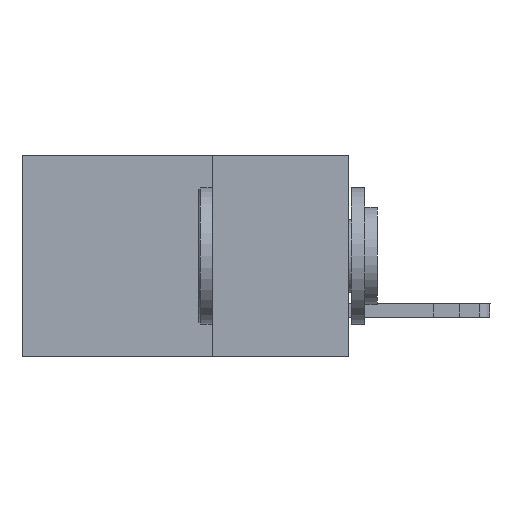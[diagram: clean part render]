
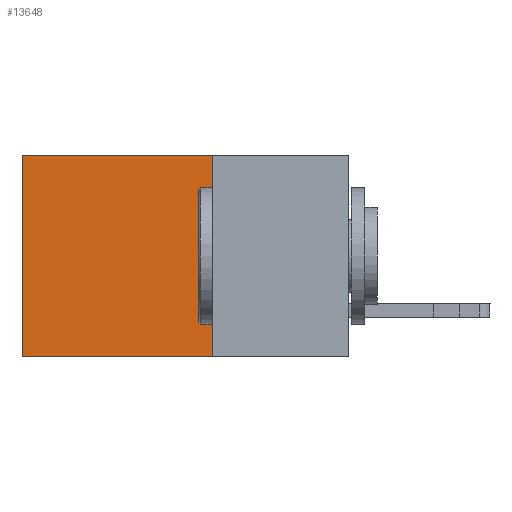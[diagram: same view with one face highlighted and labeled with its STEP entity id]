
A CAD part, left-side view. The second image highlights one B-rep face of the part: STEP entity #13648.
In plain terms, the highlighted planar face has unit normal (-1, 0, 0).
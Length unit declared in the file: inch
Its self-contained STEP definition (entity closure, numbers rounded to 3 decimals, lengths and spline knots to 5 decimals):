
#90 = VERTEX_POINT ( 'NONE', #14742 ) ;
#517 = LINE ( 'NONE', #11431, #14015 ) ;
#1959 = DIRECTION ( 'NONE',  ( 0., 0., -1. ) ) ;
#2169 = FACE_OUTER_BOUND ( 'NONE', #11980, .T. ) ;
#3057 = CARTESIAN_POINT ( 'NONE',  ( 0.298, 0.25, 0. ) ) ;
#3629 = VERTEX_POINT ( 'NONE', #11066 ) ;
#4095 = AXIS2_PLACEMENT_3D ( 'NONE', #15564, #9477, #11961 ) ;
#4279 = VECTOR ( 'NONE', #1959, 39.37008 ) ;
#5092 = VERTEX_POINT ( 'NONE', #12670 ) ;
#5637 = CARTESIAN_POINT ( 'NONE',  ( 0.298, 0.25, -0.37 ) ) ;
#6116 = ORIENTED_EDGE ( 'NONE', *, *, #13691, .F. ) ;
#6159 = VERTEX_POINT ( 'NONE', #5637 ) ;
#7059 = PLANE ( 'NONE',  #4095 ) ;
#7241 = EDGE_CURVE ( 'NONE', #6159, #3629, #517, .T. ) ;
#7521 = DIRECTION ( 'NONE',  ( 0., 0., -1. ) ) ;
#8971 = ORIENTED_EDGE ( 'NONE', *, *, #7241, .F. ) ;
#9103 = DIRECTION ( 'NONE',  ( 0., 1., 0. ) ) ;
#9477 = DIRECTION ( 'NONE',  ( 1., 0., 0. ) ) ;
#9647 = ORIENTED_EDGE ( 'NONE', *, *, #14740, .T. ) ;
#9884 = EDGE_CURVE ( 'NONE', #90, #3629, #15367, .T. ) ;
#10474 = CARTESIAN_POINT ( 'NONE',  ( 0.298, 0.6, 0. ) ) ;
#11066 = CARTESIAN_POINT ( 'NONE',  ( 0.298, 0.6, -0.37 ) ) ;
#11431 = CARTESIAN_POINT ( 'NONE',  ( 0.298, 0.25, -0.37 ) ) ;
#11881 = DIRECTION ( 'NONE',  ( 0., 1., 0. ) ) ;
#11961 = DIRECTION ( 'NONE',  ( 0., 0., -1. ) ) ;
#11980 = EDGE_LOOP ( 'NONE', ( #12576, #8971, #6116, #9647 ) ) ;
#12508 = LINE ( 'NONE', #13483, #15358 ) ;
#12576 = ORIENTED_EDGE ( 'NONE', *, *, #9884, .T. ) ;
#12670 = CARTESIAN_POINT ( 'NONE',  ( 0.298, 0.25, 0. ) ) ;
#13350 = VECTOR ( 'NONE', #11881, 39.37008 ) ;
#13483 = CARTESIAN_POINT ( 'NONE',  ( 0.298, 0.25, 0. ) ) ;
#13648 = ADVANCED_FACE ( 'NONE', ( #2169 ), #7059, .F. ) ;
#13691 = EDGE_CURVE ( 'NONE', #5092, #6159, #12508, .T. ) ;
#14015 = VECTOR ( 'NONE', #9103, 39.37008 ) ;
#14052 = LINE ( 'NONE', #3057, #13350 ) ;
#14740 = EDGE_CURVE ( 'NONE', #5092, #90, #14052, .T. ) ;
#14742 = CARTESIAN_POINT ( 'NONE',  ( 0.298, 0.6, 0. ) ) ;
#15358 = VECTOR ( 'NONE', #7521, 39.37008 ) ;
#15367 = LINE ( 'NONE', #10474, #4279 ) ;
#15564 = CARTESIAN_POINT ( 'NONE',  ( 0.298, 0.25, 0. ) ) ;
